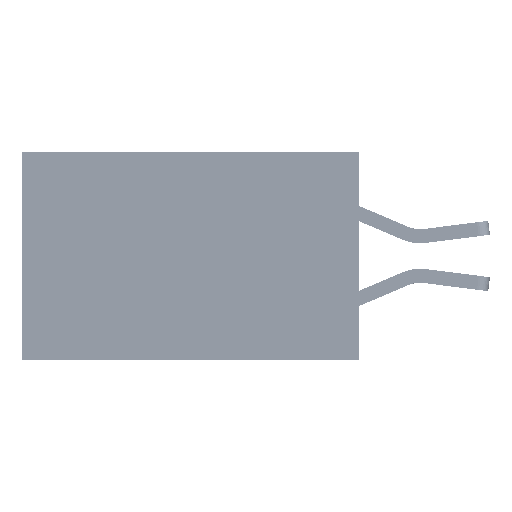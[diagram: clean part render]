
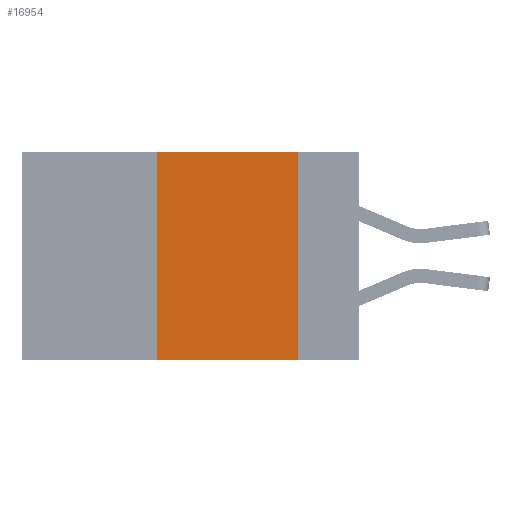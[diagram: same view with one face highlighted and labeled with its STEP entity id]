
A CAD part, left-side view. The second image highlights one B-rep face of the part: STEP entity #16954.
In plain terms, the highlighted planar face has unit normal (-1, 0, 0).
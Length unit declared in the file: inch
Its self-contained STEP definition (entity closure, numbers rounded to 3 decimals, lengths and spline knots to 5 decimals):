
#653 = VERTEX_POINT ( 'NONE', #29592 ) ;
#2653 = VERTEX_POINT ( 'NONE', #19423 ) ;
#2673 = LINE ( 'NONE', #6543, #22577 ) ;
#5570 = VECTOR ( 'NONE', #35536, 39.37008 ) ;
#5655 = VECTOR ( 'NONE', #28481, 39.37008 ) ;
#6543 = CARTESIAN_POINT ( 'NONE',  ( 0., 0.6, -0.37 ) ) ;
#7894 = EDGE_CURVE ( 'NONE', #43714, #2653, #20972, .T. ) ;
#9669 = CARTESIAN_POINT ( 'NONE',  ( 0., 0.36, 0. ) ) ;
#10043 = CARTESIAN_POINT ( 'NONE',  ( 0., 0.11, 0. ) ) ;
#10676 = CARTESIAN_POINT ( 'NONE',  ( 0., 0.6, 0. ) ) ;
#13157 = PLANE ( 'NONE',  #37660 ) ;
#13200 = ORIENTED_EDGE ( 'NONE', *, *, #28614, .T. ) ;
#14875 = VERTEX_POINT ( 'NONE', #20808 ) ;
#16954 = ADVANCED_FACE ( 'NONE', ( #42512 ), #13157, .F. ) ;
#17595 = DIRECTION ( 'NONE',  ( 0., 0., 1. ) ) ;
#18141 = LINE ( 'NONE', #10676, #5655 ) ;
#19423 = CARTESIAN_POINT ( 'NONE',  ( 0., 0.36, 0. ) ) ;
#20808 = CARTESIAN_POINT ( 'NONE',  ( 0., 0.11, -0.37 ) ) ;
#20972 = LINE ( 'NONE', #9669, #34229 ) ;
#21335 = CARTESIAN_POINT ( 'NONE',  ( 0., 0.6, 0. ) ) ;
#22577 = VECTOR ( 'NONE', #42629, 39.37008 ) ;
#25209 = EDGE_CURVE ( 'NONE', #653, #14875, #31698, .T. ) ;
#26054 = ORIENTED_EDGE ( 'NONE', *, *, #37082, .F. ) ;
#28303 = DIRECTION ( 'NONE',  ( 0., 0., -1. ) ) ;
#28481 = DIRECTION ( 'NONE',  ( 0., -1., 0. ) ) ;
#28614 = EDGE_CURVE ( 'NONE', #43714, #14875, #2673, .T. ) ;
#29592 = CARTESIAN_POINT ( 'NONE',  ( 0., 0.11, 0. ) ) ;
#31457 = DIRECTION ( 'NONE',  ( 1., 0., 0. ) ) ;
#31698 = LINE ( 'NONE', #10043, #5570 ) ;
#34229 = VECTOR ( 'NONE', #17595, 39.37008 ) ;
#35536 = DIRECTION ( 'NONE',  ( 0., 0., -1. ) ) ;
#36046 = ORIENTED_EDGE ( 'NONE', *, *, #7894, .F. ) ;
#37082 = EDGE_CURVE ( 'NONE', #2653, #653, #18141, .T. ) ;
#37660 = AXIS2_PLACEMENT_3D ( 'NONE', #21335, #31457, #28303 ) ;
#38210 = CARTESIAN_POINT ( 'NONE',  ( 0., 0.36, -0.37 ) ) ;
#40438 = ORIENTED_EDGE ( 'NONE', *, *, #25209, .F. ) ;
#41378 = EDGE_LOOP ( 'NONE', ( #40438, #26054, #36046, #13200 ) ) ;
#42512 = FACE_OUTER_BOUND ( 'NONE', #41378, .T. ) ;
#42629 = DIRECTION ( 'NONE',  ( 0., -1., 0. ) ) ;
#43714 = VERTEX_POINT ( 'NONE', #38210 ) ;
